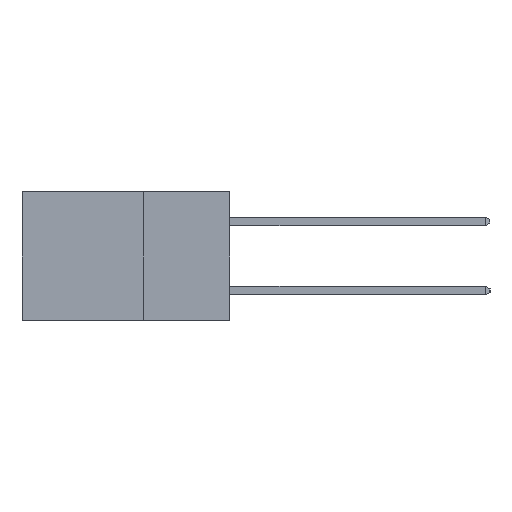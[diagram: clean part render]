
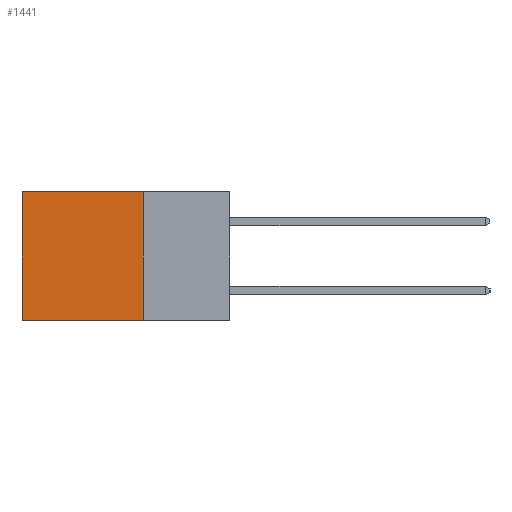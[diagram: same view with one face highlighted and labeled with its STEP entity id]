
A CAD part, left-side view. The second image highlights one B-rep face of the part: STEP entity #1441.
In plain terms, the highlighted planar face has unit normal (-1, 0, 0).
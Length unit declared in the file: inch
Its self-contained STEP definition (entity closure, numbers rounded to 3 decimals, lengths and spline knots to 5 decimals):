
#344 = EDGE_LOOP ( 'NONE', ( #6514, #12468, #471, #3966 ) ) ;
#471 = ORIENTED_EDGE ( 'NONE', *, *, #7165, .F. ) ;
#930 = EDGE_CURVE ( 'NONE', #8425, #3518, #10880, .T. ) ;
#1160 = VECTOR ( 'NONE', #9724, 39.37008 ) ;
#1441 = ADVANCED_FACE ( 'NONE', ( #10162 ), #10936, .F. ) ;
#1975 = VECTOR ( 'NONE', #12441, 39.37008 ) ;
#2681 = VECTOR ( 'NONE', #5880, 39.37008 ) ;
#3066 = LINE ( 'NONE', #5238, #2681 ) ;
#3518 = VERTEX_POINT ( 'NONE', #7573 ) ;
#3966 = ORIENTED_EDGE ( 'NONE', *, *, #13344, .T. ) ;
#5124 = LINE ( 'NONE', #13519, #1975 ) ;
#5186 = CARTESIAN_POINT ( 'NONE',  ( 0.2615, 0.25, 0. ) ) ;
#5238 = CARTESIAN_POINT ( 'NONE',  ( 0.2615, 0.25, -0.37 ) ) ;
#5486 = VECTOR ( 'NONE', #13413, 39.37008 ) ;
#5880 = DIRECTION ( 'NONE',  ( 0., 0., -1. ) ) ;
#6279 = CARTESIAN_POINT ( 'NONE',  ( 0.2615, 0.25, 0. ) ) ;
#6393 = EDGE_CURVE ( 'NONE', #6903, #3518, #5124, .T. ) ;
#6514 = ORIENTED_EDGE ( 'NONE', *, *, #6393, .T. ) ;
#6903 = VERTEX_POINT ( 'NONE', #11101 ) ;
#7165 = EDGE_CURVE ( 'NONE', #10278, #8425, #3066, .T. ) ;
#7442 = LINE ( 'NONE', #6279, #1160 ) ;
#7573 = CARTESIAN_POINT ( 'NONE',  ( 0.2615, 0.6, -0.37 ) ) ;
#8425 = VERTEX_POINT ( 'NONE', #12072 ) ;
#9724 = DIRECTION ( 'NONE',  ( 0., 1., 0. ) ) ;
#10162 = FACE_OUTER_BOUND ( 'NONE', #344, .T. ) ;
#10278 = VERTEX_POINT ( 'NONE', #5186 ) ;
#10790 = DIRECTION ( 'NONE',  ( 0., 0., -1. ) ) ;
#10803 = DIRECTION ( 'NONE',  ( 1., 0., 0. ) ) ;
#10880 = LINE ( 'NONE', #12211, #5486 ) ;
#10936 = PLANE ( 'NONE',  #11268 ) ;
#11018 = CARTESIAN_POINT ( 'NONE',  ( 0.2615, 0.25, -0.37 ) ) ;
#11101 = CARTESIAN_POINT ( 'NONE',  ( 0.2615, 0.6, 0. ) ) ;
#11268 = AXIS2_PLACEMENT_3D ( 'NONE', #11018, #10803, #10790 ) ;
#12072 = CARTESIAN_POINT ( 'NONE',  ( 0.2615, 0.25, -0.37 ) ) ;
#12211 = CARTESIAN_POINT ( 'NONE',  ( 0.2615, 0.25, -0.37 ) ) ;
#12441 = DIRECTION ( 'NONE',  ( 0., 0., -1. ) ) ;
#12468 = ORIENTED_EDGE ( 'NONE', *, *, #930, .F. ) ;
#13344 = EDGE_CURVE ( 'NONE', #10278, #6903, #7442, .T. ) ;
#13413 = DIRECTION ( 'NONE',  ( 0., 1., 0. ) ) ;
#13519 = CARTESIAN_POINT ( 'NONE',  ( 0.2615, 0.6, -0.37 ) ) ;
